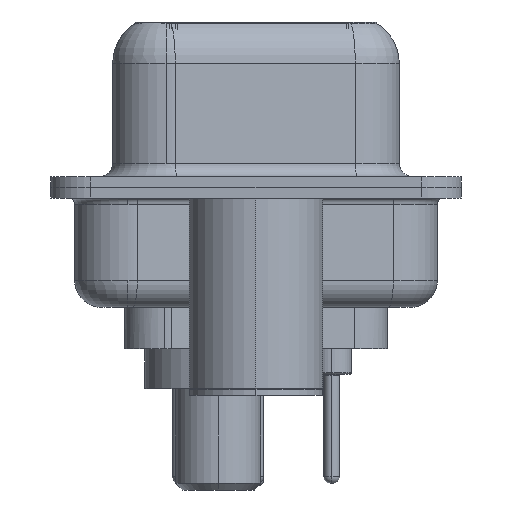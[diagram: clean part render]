
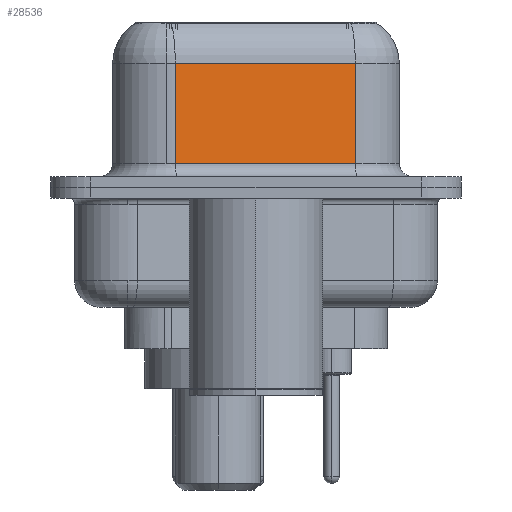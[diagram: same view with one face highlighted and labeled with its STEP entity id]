
A CAD part, left-side view. The second image highlights one B-rep face of the part: STEP entity #28536.
In plain terms, the highlighted planar face has unit normal (-0.985, -0.174, 0).
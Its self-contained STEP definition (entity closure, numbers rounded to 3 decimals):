
#1989 = VECTOR ( 'NONE', #10835, 1000. ) ;
#3697 = VERTEX_POINT ( 'NONE', #22488 ) ;
#6218 = CARTESIAN_POINT ( 'NONE',  ( 5.621, -3.722, 6.4 ) ) ;
#6258 = EDGE_LOOP ( 'NONE', ( #33986, #21399, #9866, #19641 ) ) ;
#6293 = VECTOR ( 'NONE', #22566, 1000. ) ;
#6430 = VERTEX_POINT ( 'NONE', #22373 ) ;
#7012 = VECTOR ( 'NONE', #9982, 1000. ) ;
#9866 = ORIENTED_EDGE ( 'NONE', *, *, #31832, .T. ) ;
#9982 = DIRECTION ( 'NONE',  ( 0., 0., -1. ) ) ;
#10741 = CARTESIAN_POINT ( 'NONE',  ( 5.621, -3.722, 6.4 ) ) ;
#10835 = DIRECTION ( 'NONE',  ( -0.174, 0.985, 0. ) ) ;
#10863 = PLANE ( 'NONE',  #31566 ) ;
#12358 = CARTESIAN_POINT ( 'NONE',  ( 4.43, 3.028, 0.9 ) ) ;
#12535 = CARTESIAN_POINT ( 'NONE',  ( 4.43, 3.028, 6.4 ) ) ;
#13624 = DIRECTION ( 'NONE',  ( 0.985, 0.174, 0. ) ) ;
#14082 = LINE ( 'NONE', #12535, #7012 ) ;
#16423 = VERTEX_POINT ( 'NONE', #23605 ) ;
#18155 = CARTESIAN_POINT ( 'NONE',  ( 5.621, -3.722, 4.65 ) ) ;
#19641 = ORIENTED_EDGE ( 'NONE', *, *, #28863, .T. ) ;
#20023 = VERTEX_POINT ( 'NONE', #12358 ) ;
#21399 = ORIENTED_EDGE ( 'NONE', *, *, #24690, .T. ) ;
#22067 = LINE ( 'NONE', #27654, #28247 ) ;
#22373 = CARTESIAN_POINT ( 'NONE',  ( 5.621, -3.722, 4.65 ) ) ;
#22488 = CARTESIAN_POINT ( 'NONE',  ( 4.43, 3.028, 4.65 ) ) ;
#22566 = DIRECTION ( 'NONE',  ( 0., 0., -1. ) ) ;
#23605 = CARTESIAN_POINT ( 'NONE',  ( 5.621, -3.722, 0.9 ) ) ;
#24303 = DIRECTION ( 'NONE',  ( -0.174, 0.985, 0. ) ) ;
#24690 = EDGE_CURVE ( 'NONE', #6430, #3697, #32658, .T. ) ;
#25123 = DIRECTION ( 'NONE',  ( 0.174, -0.985, 0. ) ) ;
#25377 = LINE ( 'NONE', #6218, #6293 ) ;
#27654 = CARTESIAN_POINT ( 'NONE',  ( 5.621, -3.722, 0.9 ) ) ;
#28247 = VECTOR ( 'NONE', #25123, 1000. ) ;
#28536 = ADVANCED_FACE ( 'NONE', ( #33228 ), #10863, .F. ) ;
#28756 = EDGE_CURVE ( 'NONE', #6430, #16423, #25377, .T. ) ;
#28863 = EDGE_CURVE ( 'NONE', #20023, #16423, #22067, .T. ) ;
#31566 = AXIS2_PLACEMENT_3D ( 'NONE', #10741, #13624, #24303 ) ;
#31832 = EDGE_CURVE ( 'NONE', #3697, #20023, #14082, .T. ) ;
#32658 = LINE ( 'NONE', #18155, #1989 ) ;
#33228 = FACE_OUTER_BOUND ( 'NONE', #6258, .T. ) ;
#33986 = ORIENTED_EDGE ( 'NONE', *, *, #28756, .F. ) ;
